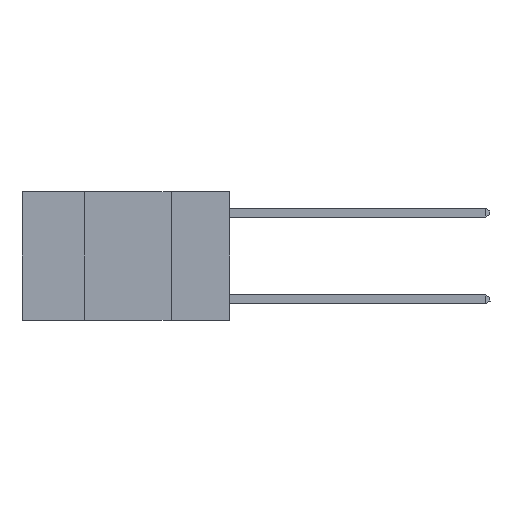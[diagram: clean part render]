
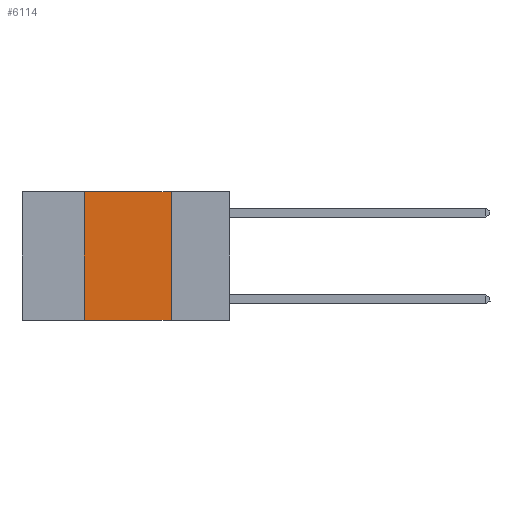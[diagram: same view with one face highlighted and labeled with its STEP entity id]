
A CAD part, left-side view. The second image highlights one B-rep face of the part: STEP entity #6114.
In plain terms, the highlighted planar face has unit normal (-1, 0, 0).
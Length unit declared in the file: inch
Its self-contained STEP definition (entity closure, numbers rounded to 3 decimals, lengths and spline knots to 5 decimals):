
#608 = LINE ( 'NONE', #10877, #2931 ) ;
#725 = CARTESIAN_POINT ( 'NONE',  ( 0., 0.17, -0.37 ) ) ;
#938 = VERTEX_POINT ( 'NONE', #5609 ) ;
#1554 = VECTOR ( 'NONE', #9378, 39.37008 ) ;
#1726 = CARTESIAN_POINT ( 'NONE',  ( 0., 0.42, 0. ) ) ;
#1757 = DIRECTION ( 'NONE',  ( 1., 0., 0. ) ) ;
#1810 = ORIENTED_EDGE ( 'NONE', *, *, #10188, .F. ) ;
#2050 = LINE ( 'NONE', #8477, #10518 ) ;
#2066 = CARTESIAN_POINT ( 'NONE',  ( 0., 0.17, 0. ) ) ;
#2215 = AXIS2_PLACEMENT_3D ( 'NONE', #5164, #1757, #7748 ) ;
#2454 = DIRECTION ( 'NONE',  ( 0., 0., -1. ) ) ;
#2530 = DIRECTION ( 'NONE',  ( 0., -1., 0. ) ) ;
#2931 = VECTOR ( 'NONE', #5023, 39.37008 ) ;
#2938 = ORIENTED_EDGE ( 'NONE', *, *, #8533, .F. ) ;
#2978 = VERTEX_POINT ( 'NONE', #725 ) ;
#4461 = ORIENTED_EDGE ( 'NONE', *, *, #10249, .F. ) ;
#5023 = DIRECTION ( 'NONE',  ( 0., -1., 0. ) ) ;
#5164 = CARTESIAN_POINT ( 'NONE',  ( 0., 0.6, 0. ) ) ;
#5609 = CARTESIAN_POINT ( 'NONE',  ( 0., 0.42, 0. ) ) ;
#6114 = ADVANCED_FACE ( 'NONE', ( #8543 ), #6874, .F. ) ;
#6367 = LINE ( 'NONE', #1726, #1554 ) ;
#6874 = PLANE ( 'NONE',  #2215 ) ;
#7139 = LINE ( 'NONE', #8410, #9111 ) ;
#7165 = VERTEX_POINT ( 'NONE', #9855 ) ;
#7748 = DIRECTION ( 'NONE',  ( 0., 0., -1. ) ) ;
#7986 = EDGE_CURVE ( 'NONE', #7165, #2978, #608, .T. ) ;
#8151 = ORIENTED_EDGE ( 'NONE', *, *, #7986, .T. ) ;
#8410 = CARTESIAN_POINT ( 'NONE',  ( 0., 0.17, 0. ) ) ;
#8477 = CARTESIAN_POINT ( 'NONE',  ( 0., 0.6, 0. ) ) ;
#8533 = EDGE_CURVE ( 'NONE', #7165, #938, #6367, .T. ) ;
#8543 = FACE_OUTER_BOUND ( 'NONE', #10045, .T. ) ;
#8760 = VERTEX_POINT ( 'NONE', #2066 ) ;
#9111 = VECTOR ( 'NONE', #2454, 39.37008 ) ;
#9378 = DIRECTION ( 'NONE',  ( 0., 0., 1. ) ) ;
#9855 = CARTESIAN_POINT ( 'NONE',  ( 0., 0.42, -0.37 ) ) ;
#10045 = EDGE_LOOP ( 'NONE', ( #1810, #4461, #2938, #8151 ) ) ;
#10188 = EDGE_CURVE ( 'NONE', #8760, #2978, #7139, .T. ) ;
#10249 = EDGE_CURVE ( 'NONE', #938, #8760, #2050, .T. ) ;
#10518 = VECTOR ( 'NONE', #2530, 39.37008 ) ;
#10877 = CARTESIAN_POINT ( 'NONE',  ( 0., 0.6, -0.37 ) ) ;
